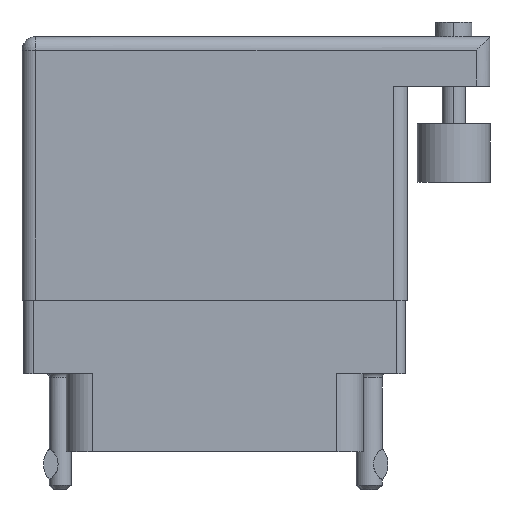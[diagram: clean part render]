
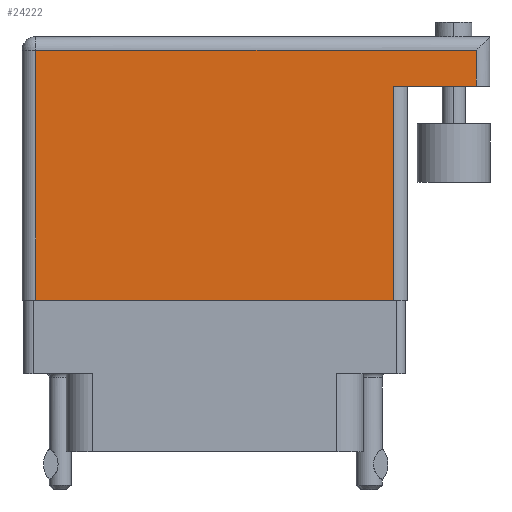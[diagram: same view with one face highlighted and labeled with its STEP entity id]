
A CAD part, front view. The second image highlights one B-rep face of the part: STEP entity #24222.
In plain terms, the highlighted face is planar.
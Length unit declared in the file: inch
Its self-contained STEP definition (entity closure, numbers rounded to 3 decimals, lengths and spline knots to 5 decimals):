
#2581 = CARTESIAN_POINT ( 'NONE',  ( 1.278, 0.736, 0. ) ) ;
#2823 = CARTESIAN_POINT ( 'NONE',  ( 1.278, 0., 0. ) ) ;
#3997 = VECTOR ( 'NONE', #29664, 39.37008 ) ;
#4372 = EDGE_CURVE ( 'NONE', #34678, #8876, #21212, .T. ) ;
#4380 = VERTEX_POINT ( 'NONE', #10362 ) ;
#4593 = LINE ( 'NONE', #22443, #24812 ) ;
#5764 = VECTOR ( 'NONE', #33509, 39.37008 ) ;
#5949 = CARTESIAN_POINT ( 'NONE',  ( 0., 0.906, 0. ) ) ;
#8876 = VERTEX_POINT ( 'NONE', #15631 ) ;
#9776 = DIRECTION ( 'NONE',  ( 0., -1., 0. ) ) ;
#10362 = CARTESIAN_POINT ( 'NONE',  ( 1.562, 0.736, 0. ) ) ;
#10583 = VECTOR ( 'NONE', #16414, 39.37008 ) ;
#10870 = CARTESIAN_POINT ( 'NONE',  ( 1.562, 0.906, 0. ) ) ;
#10984 = ORIENTED_EDGE ( 'NONE', *, *, #29931, .T. ) ;
#11332 = LINE ( 'NONE', #26689, #3997 ) ;
#11889 = FACE_OUTER_BOUND ( 'NONE', #19990, .T. ) ;
#11959 = VERTEX_POINT ( 'NONE', #22430 ) ;
#12316 = VERTEX_POINT ( 'NONE', #31403 ) ;
#14075 = EDGE_CURVE ( 'NONE', #4380, #11959, #11332, .T. ) ;
#14386 = DIRECTION ( 'NONE',  ( 1., 0., 0. ) ) ;
#14399 = LINE ( 'NONE', #2581, #32002 ) ;
#15631 = CARTESIAN_POINT ( 'NONE',  ( 0.047, 0., 0. ) ) ;
#16414 = DIRECTION ( 'NONE',  ( 0., 1., 0. ) ) ;
#16788 = PLANE ( 'NONE',  #30022 ) ;
#16969 = ORIENTED_EDGE ( 'NONE', *, *, #24307, .T. ) ;
#17247 = ORIENTED_EDGE ( 'NONE', *, *, #14075, .F. ) ;
#18119 = ORIENTED_EDGE ( 'NONE', *, *, #30863, .T. ) ;
#19196 = DIRECTION ( 'NONE',  ( 0., 1., 0. ) ) ;
#19990 = EDGE_LOOP ( 'NONE', ( #16969, #29260, #17247, #10984, #18119, #31410 ) ) ;
#20474 = LINE ( 'NONE', #10870, #10583 ) ;
#21212 = LINE ( 'NONE', #34426, #22070 ) ;
#22070 = VECTOR ( 'NONE', #9776, 39.37008 ) ;
#22430 = CARTESIAN_POINT ( 'NONE',  ( 1.278, 0.736, 0. ) ) ;
#22443 = CARTESIAN_POINT ( 'NONE',  ( 0., 0., 0. ) ) ;
#22743 = VERTEX_POINT ( 'NONE', #2823 ) ;
#23472 = CARTESIAN_POINT ( 'NONE',  ( 0.047, 0.859, 0. ) ) ;
#24222 = ADVANCED_FACE ( 'NONE', ( #11889 ), #16788, .F. ) ;
#24307 = EDGE_CURVE ( 'NONE', #8876, #22743, #4593, .T. ) ;
#24812 = VECTOR ( 'NONE', #14386, 39.37008 ) ;
#26007 = LINE ( 'NONE', #31220, #5764 ) ;
#26689 = CARTESIAN_POINT ( 'NONE',  ( 1.609, 0.736, 0. ) ) ;
#27203 = EDGE_CURVE ( 'NONE', #22743, #11959, #14399, .T. ) ;
#29260 = ORIENTED_EDGE ( 'NONE', *, *, #27203, .T. ) ;
#29664 = DIRECTION ( 'NONE',  ( -1., 0., 0. ) ) ;
#29931 = EDGE_CURVE ( 'NONE', #4380, #12316, #20474, .T. ) ;
#30022 = AXIS2_PLACEMENT_3D ( 'NONE', #5949, #30705, #33376 ) ;
#30705 = DIRECTION ( 'NONE',  ( 0., 0., -1. ) ) ;
#30863 = EDGE_CURVE ( 'NONE', #12316, #34678, #26007, .T. ) ;
#31220 = CARTESIAN_POINT ( 'NONE',  ( 0., 0.859, 0. ) ) ;
#31403 = CARTESIAN_POINT ( 'NONE',  ( 1.562, 0.859, 0. ) ) ;
#31410 = ORIENTED_EDGE ( 'NONE', *, *, #4372, .T. ) ;
#32002 = VECTOR ( 'NONE', #19196, 39.37008 ) ;
#33376 = DIRECTION ( 'NONE',  ( -1., 0., 0. ) ) ;
#33509 = DIRECTION ( 'NONE',  ( -1., 0., 0. ) ) ;
#34426 = CARTESIAN_POINT ( 'NONE',  ( 0.047, 0., 0. ) ) ;
#34678 = VERTEX_POINT ( 'NONE', #23472 ) ;
